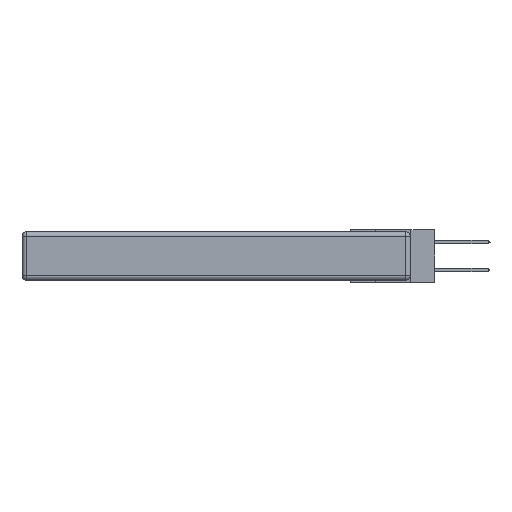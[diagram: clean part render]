
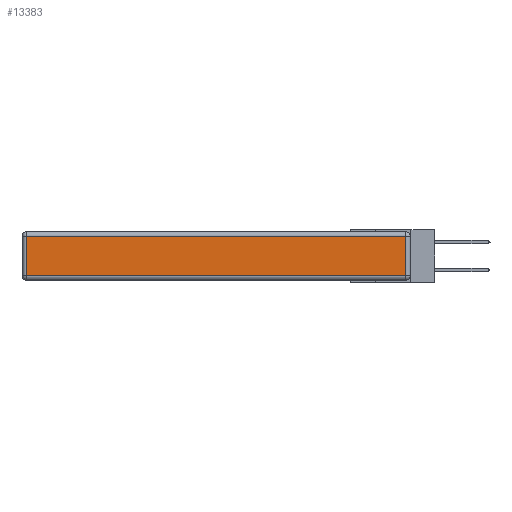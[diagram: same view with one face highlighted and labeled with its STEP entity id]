
A CAD part, left-side view. The second image highlights one B-rep face of the part: STEP entity #13383.
In plain terms, the highlighted planar face has unit normal (-1, 0, 0).
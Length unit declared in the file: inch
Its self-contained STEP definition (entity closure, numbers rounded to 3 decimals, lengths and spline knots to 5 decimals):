
#283 = DIRECTION ( 'NONE',  ( 0., 0., 1. ) ) ;
#586 = VERTEX_POINT ( 'NONE', #25145 ) ;
#726 = CARTESIAN_POINT ( 'NONE',  ( 0., 2.72, -0.313 ) ) ;
#2401 = LINE ( 'NONE', #19455, #28376 ) ;
#2753 = CARTESIAN_POINT ( 'NONE',  ( 0., 0.03, -0.313 ) ) ;
#3117 = CARTESIAN_POINT ( 'NONE',  ( 0., 2.72, -0.03 ) ) ;
#3922 = VERTEX_POINT ( 'NONE', #726 ) ;
#5174 = EDGE_CURVE ( 'NONE', #3922, #15255, #23870, .T. ) ;
#5805 = ORIENTED_EDGE ( 'NONE', *, *, #6168, .T. ) ;
#6168 = EDGE_CURVE ( 'NONE', #15255, #586, #27479, .T. ) ;
#7992 = CARTESIAN_POINT ( 'NONE',  ( 0., 0., -0.343 ) ) ;
#10406 = AXIS2_PLACEMENT_3D ( 'NONE', #7992, #26372, #283 ) ;
#10740 = VECTOR ( 'NONE', #14664, 39.37008 ) ;
#10748 = EDGE_LOOP ( 'NONE', ( #12367, #5805, #23773, #30637 ) ) ;
#11265 = CARTESIAN_POINT ( 'NONE',  ( 0., 0.03, -0.343 ) ) ;
#12367 = ORIENTED_EDGE ( 'NONE', *, *, #5174, .T. ) ;
#13383 = ADVANCED_FACE ( 'NONE', ( #24167 ), #23446, .T. ) ;
#14664 = DIRECTION ( 'NONE',  ( 0., 1., 0. ) ) ;
#14815 = LINE ( 'NONE', #18176, #10740 ) ;
#15255 = VERTEX_POINT ( 'NONE', #2753 ) ;
#16110 = VECTOR ( 'NONE', #24259, 39.37008 ) ;
#17768 = VERTEX_POINT ( 'NONE', #3117 ) ;
#18142 = EDGE_CURVE ( 'NONE', #17768, #3922, #2401, .T. ) ;
#18176 = CARTESIAN_POINT ( 'NONE',  ( 0., 2.75, -0.03 ) ) ;
#19455 = CARTESIAN_POINT ( 'NONE',  ( 0., 2.72, -0.343 ) ) ;
#19991 = EDGE_CURVE ( 'NONE', #586, #17768, #14815, .T. ) ;
#21636 = CARTESIAN_POINT ( 'NONE',  ( 0., 0., -0.313 ) ) ;
#21903 = DIRECTION ( 'NONE',  ( 0., 0., 1. ) ) ;
#23446 = PLANE ( 'NONE',  #10406 ) ;
#23773 = ORIENTED_EDGE ( 'NONE', *, *, #19991, .T. ) ;
#23870 = LINE ( 'NONE', #21636, #16110 ) ;
#24167 = FACE_OUTER_BOUND ( 'NONE', #10748, .T. ) ;
#24259 = DIRECTION ( 'NONE',  ( 0., -1., 0. ) ) ;
#24682 = DIRECTION ( 'NONE',  ( 0., 0., -1. ) ) ;
#25145 = CARTESIAN_POINT ( 'NONE',  ( 0., 0.03, -0.03 ) ) ;
#26372 = DIRECTION ( 'NONE',  ( -1., 0., 0. ) ) ;
#27479 = LINE ( 'NONE', #11265, #32315 ) ;
#28376 = VECTOR ( 'NONE', #24682, 39.37008 ) ;
#30637 = ORIENTED_EDGE ( 'NONE', *, *, #18142, .T. ) ;
#32315 = VECTOR ( 'NONE', #21903, 39.37008 ) ;
